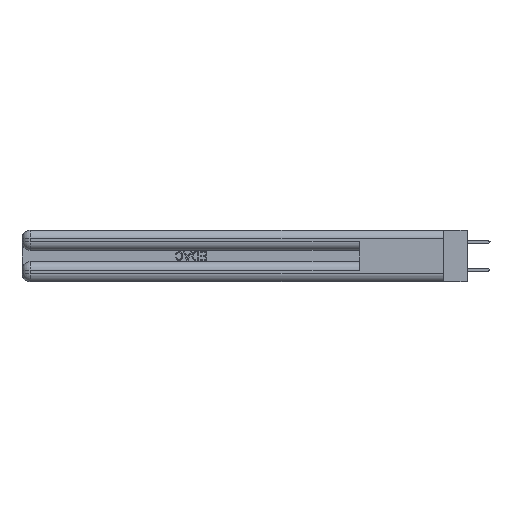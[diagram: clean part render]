
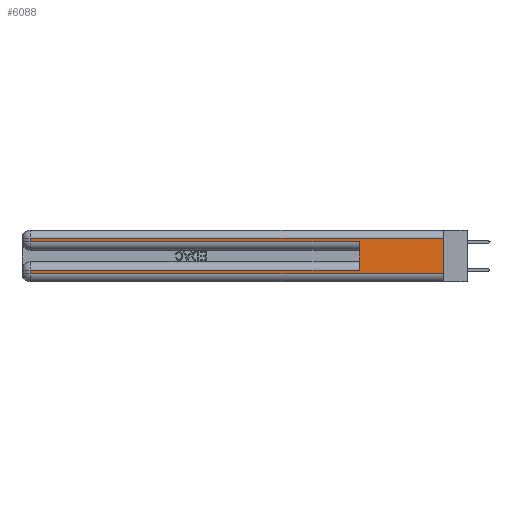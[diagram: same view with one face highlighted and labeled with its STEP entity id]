
A CAD part, left-side view. The second image highlights one B-rep face of the part: STEP entity #6088.
In plain terms, the highlighted planar face has unit normal (-1, 0, 0).
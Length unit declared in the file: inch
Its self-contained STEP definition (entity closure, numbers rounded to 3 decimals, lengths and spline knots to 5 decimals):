
#411 = CARTESIAN_POINT ( 'NONE',  ( 0., 0., 0.37 ) ) ;
#1056 = DIRECTION ( 'NONE',  ( 0., 0., -1. ) ) ;
#1706 = CARTESIAN_POINT ( 'NONE',  ( 0., 0.6, 0.285 ) ) ;
#1709 = VERTEX_POINT ( 'NONE', #26420 ) ;
#2831 = ORIENTED_EDGE ( 'NONE', *, *, #12281, .F. ) ;
#3945 = CARTESIAN_POINT ( 'NONE',  ( 0., 2.94, 0.285 ) ) ;
#6088 = ADVANCED_FACE ( 'NONE', ( #28569 ), #14295, .F. ) ;
#6122 = ORIENTED_EDGE ( 'NONE', *, *, #41387, .T. ) ;
#6140 = LINE ( 'NONE', #13686, #39881 ) ;
#7075 = ORIENTED_EDGE ( 'NONE', *, *, #11564, .T. ) ;
#8239 = AXIS2_PLACEMENT_3D ( 'NONE', #31624, #35252, #34799 ) ;
#9170 = LINE ( 'NONE', #31755, #15622 ) ;
#9499 = VERTEX_POINT ( 'NONE', #22385 ) ;
#11564 = EDGE_CURVE ( 'NONE', #1709, #41519, #23809, .T. ) ;
#12281 = EDGE_CURVE ( 'NONE', #13362, #9499, #26833, .T. ) ;
#12547 = DIRECTION ( 'NONE',  ( 0., 0., 1. ) ) ;
#13066 = EDGE_CURVE ( 'NONE', #13362, #1709, #9170, .T. ) ;
#13362 = VERTEX_POINT ( 'NONE', #39251 ) ;
#13686 = CARTESIAN_POINT ( 'NONE',  ( 0., 0., 0.085 ) ) ;
#14295 = PLANE ( 'NONE',  #8239 ) ;
#15184 = VECTOR ( 'NONE', #12547, 39.37008 ) ;
#15622 = VECTOR ( 'NONE', #24605, 39.37008 ) ;
#17308 = EDGE_CURVE ( 'NONE', #23565, #39841, #27427, .T. ) ;
#19297 = CARTESIAN_POINT ( 'NONE',  ( 0., 0.6, 0.145 ) ) ;
#19608 = ORIENTED_EDGE ( 'NONE', *, *, #44028, .T. ) ;
#20811 = ORIENTED_EDGE ( 'NONE', *, *, #36645, .T. ) ;
#21149 = LINE ( 'NONE', #40025, #36137 ) ;
#21724 = CARTESIAN_POINT ( 'NONE',  ( 0., 2.94, 0.085 ) ) ;
#22244 = CARTESIAN_POINT ( 'NONE',  ( 0., 2.94, 0.06 ) ) ;
#22385 = CARTESIAN_POINT ( 'NONE',  ( 0., 0., 0.06 ) ) ;
#23565 = VERTEX_POINT ( 'NONE', #34851 ) ;
#23809 = LINE ( 'NONE', #28013, #40926 ) ;
#24605 = DIRECTION ( 'NONE',  ( 0., 1., 0. ) ) ;
#24815 = EDGE_LOOP ( 'NONE', ( #2831, #29177, #7075, #20811, #43407, #19608, #36852, #6122 ) ) ;
#26266 = LINE ( 'NONE', #31701, #29445 ) ;
#26420 = CARTESIAN_POINT ( 'NONE',  ( 0., 2.94, 0.31 ) ) ;
#26716 = EDGE_CURVE ( 'NONE', #36546, #41131, #21149, .T. ) ;
#26833 = LINE ( 'NONE', #411, #36011 ) ;
#27106 = DIRECTION ( 'NONE',  ( 0., 1., 0. ) ) ;
#27427 = LINE ( 'NONE', #19297, #15184 ) ;
#28013 = CARTESIAN_POINT ( 'NONE',  ( 0., 2.94, 0.37 ) ) ;
#28569 = FACE_OUTER_BOUND ( 'NONE', #24815, .T. ) ;
#29177 = ORIENTED_EDGE ( 'NONE', *, *, #13066, .T. ) ;
#29445 = VECTOR ( 'NONE', #32278, 39.37008 ) ;
#29475 = DIRECTION ( 'NONE',  ( 0., 0., -1. ) ) ;
#31624 = CARTESIAN_POINT ( 'NONE',  ( 0., 0., 0.37 ) ) ;
#31701 = CARTESIAN_POINT ( 'NONE',  ( 0., 0., 0.285 ) ) ;
#31755 = CARTESIAN_POINT ( 'NONE',  ( 0., 0., 0.31 ) ) ;
#32278 = DIRECTION ( 'NONE',  ( 0., -1., 0. ) ) ;
#33830 = DIRECTION ( 'NONE',  ( 0., -1., 0. ) ) ;
#34624 = DIRECTION ( 'NONE',  ( 0., 0., -1. ) ) ;
#34799 = DIRECTION ( 'NONE',  ( 0., 0., -1. ) ) ;
#34851 = CARTESIAN_POINT ( 'NONE',  ( 0., 0.6, 0.085 ) ) ;
#35252 = DIRECTION ( 'NONE',  ( 1., 0., 0. ) ) ;
#35318 = VECTOR ( 'NONE', #33830, 39.37008 ) ;
#36011 = VECTOR ( 'NONE', #34624, 39.37008 ) ;
#36137 = VECTOR ( 'NONE', #29475, 39.37008 ) ;
#36546 = VERTEX_POINT ( 'NONE', #21724 ) ;
#36645 = EDGE_CURVE ( 'NONE', #41519, #39841, #26266, .T. ) ;
#36852 = ORIENTED_EDGE ( 'NONE', *, *, #26716, .T. ) ;
#37764 = CARTESIAN_POINT ( 'NONE',  ( 0., 0., 0.06 ) ) ;
#39251 = CARTESIAN_POINT ( 'NONE',  ( 0., 0., 0.31 ) ) ;
#39841 = VERTEX_POINT ( 'NONE', #1706 ) ;
#39881 = VECTOR ( 'NONE', #27106, 39.37008 ) ;
#40025 = CARTESIAN_POINT ( 'NONE',  ( 0., 2.94, 0.37 ) ) ;
#40926 = VECTOR ( 'NONE', #1056, 39.37008 ) ;
#41131 = VERTEX_POINT ( 'NONE', #22244 ) ;
#41387 = EDGE_CURVE ( 'NONE', #41131, #9499, #42769, .T. ) ;
#41519 = VERTEX_POINT ( 'NONE', #3945 ) ;
#42769 = LINE ( 'NONE', #37764, #35318 ) ;
#43407 = ORIENTED_EDGE ( 'NONE', *, *, #17308, .F. ) ;
#44028 = EDGE_CURVE ( 'NONE', #23565, #36546, #6140, .T. ) ;
